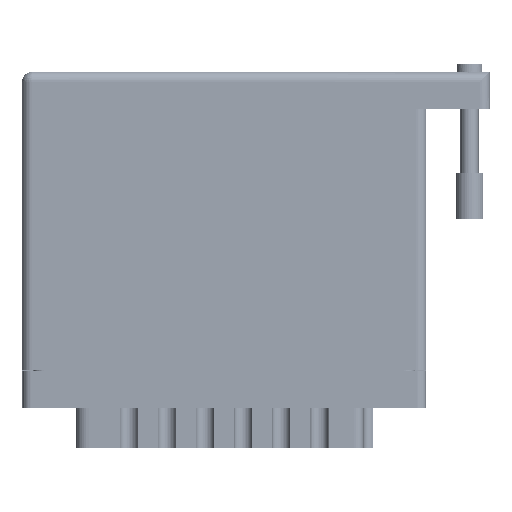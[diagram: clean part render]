
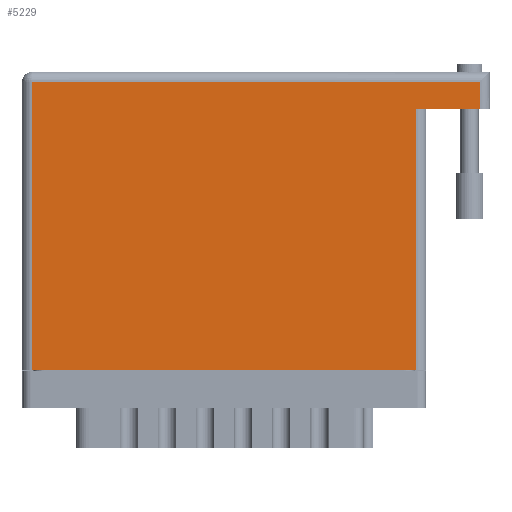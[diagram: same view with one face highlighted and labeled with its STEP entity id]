
A CAD part, front view. The second image highlights one B-rep face of the part: STEP entity #5229.
In plain terms, the highlighted face is planar.
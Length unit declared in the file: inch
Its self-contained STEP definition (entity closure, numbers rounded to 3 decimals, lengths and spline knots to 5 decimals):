
#908 = LINE ( 'NONE', #81282, #40146 ) ;
#2220 = LINE ( 'NONE', #60467, #44826 ) ;
#3191 = PLANE ( 'NONE',  #10838 ) ;
#5229 = ADVANCED_FACE ( 'NONE', ( #40026 ), #3191, .F. ) ;
#6519 = ORIENTED_EDGE ( 'NONE', *, *, #17224, .F. ) ;
#7844 = EDGE_LOOP ( 'NONE', ( #81108, #16575, #6519, #18623, #17997, #87482 ) ) ;
#8108 = CARTESIAN_POINT ( 'NONE',  ( 2.685, 0., 0. ) ) ;
#10838 = AXIS2_PLACEMENT_3D ( 'NONE', #46409, #17311, #39495 ) ;
#12131 = EDGE_CURVE ( 'NONE', #54947, #23161, #71605, .T. ) ;
#15053 = CARTESIAN_POINT ( 'NONE',  ( 0.07, 0., 0. ) ) ;
#16002 = VECTOR ( 'NONE', #22905, 39.37008 ) ;
#16575 = ORIENTED_EDGE ( 'NONE', *, *, #68808, .T. ) ;
#17103 = DIRECTION ( 'NONE',  ( 0., -1., 0. ) ) ;
#17224 = EDGE_CURVE ( 'NONE', #54947, #69387, #34247, .T. ) ;
#17311 = DIRECTION ( 'NONE',  ( 0., 0., -1. ) ) ;
#17997 = ORIENTED_EDGE ( 'NONE', *, *, #72260, .T. ) ;
#18623 = ORIENTED_EDGE ( 'NONE', *, *, #12131, .T. ) ;
#22905 = DIRECTION ( 'NONE',  ( 1., 0., 0. ) ) ;
#23161 = VERTEX_POINT ( 'NONE', #35996 ) ;
#24036 = CARTESIAN_POINT ( 'NONE',  ( 2.685, 1.774, 0. ) ) ;
#25766 = CARTESIAN_POINT ( 'NONE',  ( 0., 1.96, 0. ) ) ;
#26226 = VECTOR ( 'NONE', #75895, 39.37008 ) ;
#28041 = DIRECTION ( 'NONE',  ( -1., 0., 0. ) ) ;
#30102 = CARTESIAN_POINT ( 'NONE',  ( 0., 0., 0. ) ) ;
#32964 = LINE ( 'NONE', #25766, #26226 ) ;
#33159 = VECTOR ( 'NONE', #28041, 39.37008 ) ;
#33560 = CARTESIAN_POINT ( 'NONE',  ( 3.12, 2.03, 0. ) ) ;
#33927 = EDGE_CURVE ( 'NONE', #77738, #36916, #908, .T. ) ;
#34247 = LINE ( 'NONE', #54978, #33159 ) ;
#35996 = CARTESIAN_POINT ( 'NONE',  ( 3.12, 1.96, 0. ) ) ;
#36916 = VERTEX_POINT ( 'NONE', #15053 ) ;
#39495 = DIRECTION ( 'NONE',  ( -1., 0., 0. ) ) ;
#40026 = FACE_OUTER_BOUND ( 'NONE', #7844, .T. ) ;
#40146 = VECTOR ( 'NONE', #17103, 39.37008 ) ;
#44826 = VECTOR ( 'NONE', #89568, 39.37008 ) ;
#46409 = CARTESIAN_POINT ( 'NONE',  ( 0., 2.03, 0. ) ) ;
#49880 = EDGE_CURVE ( 'NONE', #36916, #83167, #59681, .T. ) ;
#54947 = VERTEX_POINT ( 'NONE', #82187 ) ;
#54978 = CARTESIAN_POINT ( 'NONE',  ( 3.19, 1.774, 0. ) ) ;
#56902 = CARTESIAN_POINT ( 'NONE',  ( 0.07, 1.96, 0. ) ) ;
#59681 = LINE ( 'NONE', #30102, #16002 ) ;
#60467 = CARTESIAN_POINT ( 'NONE',  ( 2.685, 1.774, 0. ) ) ;
#61517 = VECTOR ( 'NONE', #83369, 39.37008 ) ;
#68808 = EDGE_CURVE ( 'NONE', #83167, #69387, #2220, .T. ) ;
#69387 = VERTEX_POINT ( 'NONE', #24036 ) ;
#71605 = LINE ( 'NONE', #33560, #61517 ) ;
#72260 = EDGE_CURVE ( 'NONE', #23161, #77738, #32964, .T. ) ;
#75895 = DIRECTION ( 'NONE',  ( -1., 0., 0. ) ) ;
#77738 = VERTEX_POINT ( 'NONE', #56902 ) ;
#81108 = ORIENTED_EDGE ( 'NONE', *, *, #49880, .T. ) ;
#81282 = CARTESIAN_POINT ( 'NONE',  ( 0.07, 0., 0. ) ) ;
#82187 = CARTESIAN_POINT ( 'NONE',  ( 3.12, 1.774, 0. ) ) ;
#83167 = VERTEX_POINT ( 'NONE', #8108 ) ;
#83369 = DIRECTION ( 'NONE',  ( 0., 1., 0. ) ) ;
#87482 = ORIENTED_EDGE ( 'NONE', *, *, #33927, .T. ) ;
#89568 = DIRECTION ( 'NONE',  ( 0., 1., 0. ) ) ;
